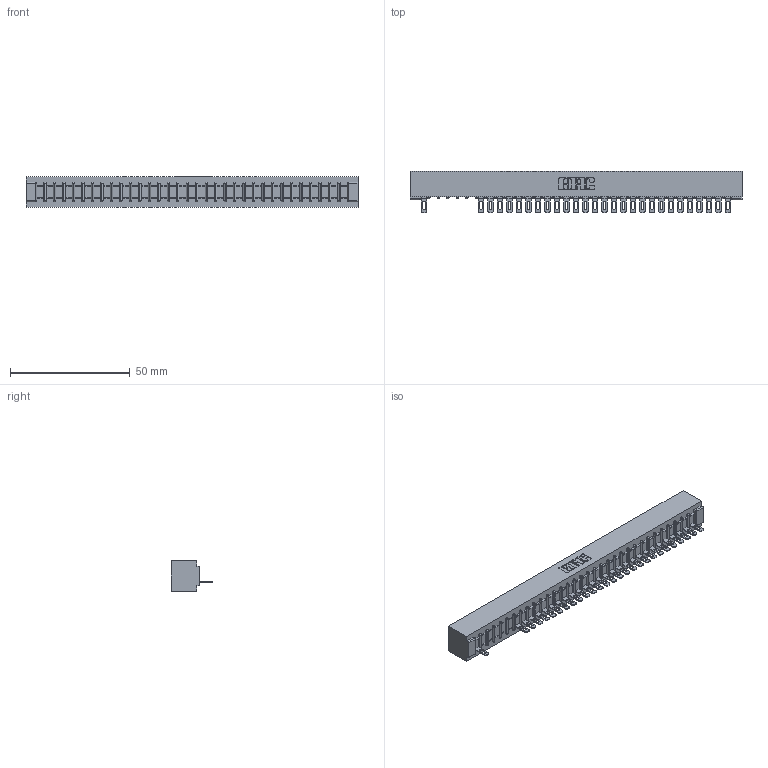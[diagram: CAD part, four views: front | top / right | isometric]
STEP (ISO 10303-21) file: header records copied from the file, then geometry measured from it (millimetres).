
FILE_DESCRIPTION (( 'STEP AP203' ), '1' );
FILE_NAME ('357-033-501-101.STEP', '2018-08-10T01:18:37', ( '' ), ( '' ), 'SwSTEP 2.0', 'SolidWorks 2016', '' );
FILE_SCHEMA (( 'CONFIG_CONTROL_DESIGN' ));
Length unit declared in the file: inch
Products named in the file (3): 307 Part_No Mounting Lugs; 307-290-002_501; 357-033-501-101
Assembly tree (29 placements, depth 2):
  357-033-501-101
    307 Part_No Mounting Lugs
    307-290-002_501  x28
Bounding box: 138.63 x 17.42 x 12.7 mm (x, y, z)
Volume: 15205.9 mm3; surface area: 18534.2 mm2
Topology: 29 solids, 29 shells, 2372 faces, 7283 edges, 4762 vertices
Faces by surface type: plane 1358, cylinder 946, sphere 68
Entity records: 29756 total; most frequent: CARTESIAN_POINT 5039, ORIENTED_EDGE 5034, DIRECTION 4897, EDGE_CURVE 2517, LINE 1921, VECTOR 1921, VERTEX_POINT 1630, AXIS2_PLACEMENT_3D 1488
